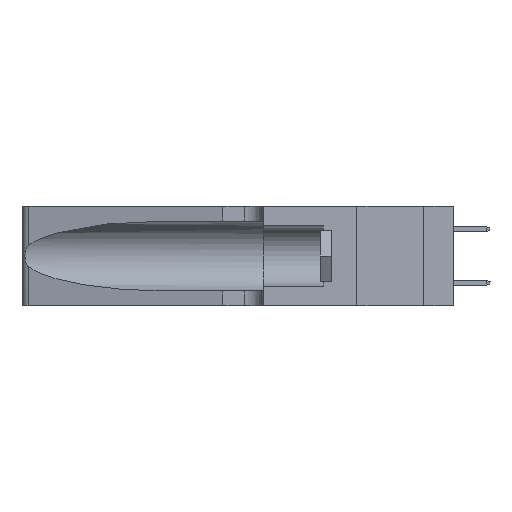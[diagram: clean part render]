
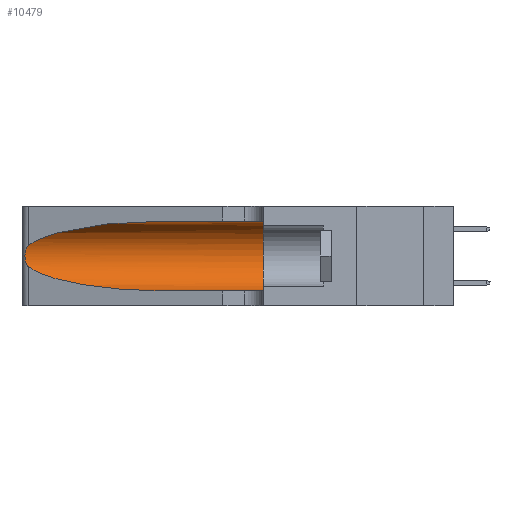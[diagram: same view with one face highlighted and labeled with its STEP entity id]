
A CAD part, left-side view. The second image highlights one B-rep face of the part: STEP entity #10479.
In plain terms, the highlighted cylindrical face has radius 3.308 mm (diameter 6.617 mm), a partial arc.
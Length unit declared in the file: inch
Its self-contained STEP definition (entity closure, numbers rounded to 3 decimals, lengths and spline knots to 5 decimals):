
#151 = CARTESIAN_POINT ( 'NONE',  ( 0.25789, 1.23486, 0.15765 ) ) ;
#358 = CYLINDRICAL_SURFACE ( 'NONE', #23111, 0.13025 ) ;
#1405 = CARTESIAN_POINT ( 'NONE',  ( 0.26018, 1.23835, 0.19895 ) ) ;
#1542 = CARTESIAN_POINT ( 'NONE',  ( 0.26017, 1.23833, 0.17102 ) ) ;
#2279 = CARTESIAN_POINT ( 'NONE',  ( 0.2373, 1.15595, 0.08982 ) ) ;
#2814 = DIRECTION ( 'NONE',  ( 0., -1., 0. ) ) ;
#2827 = CARTESIAN_POINT ( 'NONE',  ( 0.1305, 0.72297, 0.05475 ) ) ;
#3332 =( BOUNDED_CURVE ( )  B_SPLINE_CURVE ( 3, ( #8918, #2279, #21794, #2827 ),
 .UNSPECIFIED., .F., .T. ) 
 B_SPLINE_CURVE_WITH_KNOTS ( ( 4, 4 ),
 ( 3.44316, 4.71239 ),
 .UNSPECIFIED. ) 
 CURVE ( )  GEOMETRIC_REPRESENTATION_ITEM ( )  RATIONAL_B_SPLINE_CURVE ( ( 1., 0.87, 0.87, 1. ) ) 
 REPRESENTATION_ITEM ( '' )  );
#4428 = CARTESIAN_POINT ( 'NONE',  ( 0.25639, 1.23186, 0.15144 ) ) ;
#5728 = CARTESIAN_POINT ( 'NONE',  ( 0.1305, 0.72297, 0.31525 ) ) ;
#6187 =( BOUNDED_CURVE ( )  B_SPLINE_CURVE ( 3, ( #18186, #7313, #17913, #24366 ),
 .UNSPECIFIED., .F., .T. ) 
 B_SPLINE_CURVE_WITH_KNOTS ( ( 4, 4 ),
 ( 1.5708, 2.84003 ),
 .UNSPECIFIED. ) 
 CURVE ( )  GEOMETRIC_REPRESENTATION_ITEM ( )  RATIONAL_B_SPLINE_CURVE ( ( 1., 0.87, 0.87, 1. ) ) 
 REPRESENTATION_ITEM ( '' )  );
#6257 = CARTESIAN_POINT ( 'NONE',  ( 0.25555, 1.22994, 0.2215 ) ) ;
#6322 = B_SPLINE_CURVE_WITH_KNOTS ( 'NONE', 3,
 ( #25390, #6257, #20649, #23316, #20500, #1405, #9857, #18390, #1542, #25937, #151, #4428, #17109, #6814 ),
 .UNSPECIFIED., .F., .F.,
 ( 4, 2, 2, 2, 2, 2, 4 ),
 ( 0., 0.00027, 0.00053, 0.00107, 0.0016, 0.00187, 0.00214 ),
 .UNSPECIFIED. ) ;
#6324 = EDGE_CURVE ( 'NONE', #24706, #10597, #6322, .T. ) ;
#6612 = CARTESIAN_POINT ( 'NONE',  ( 0.1305, 1.61858, 0.185 ) ) ;
#6814 = CARTESIAN_POINT ( 'NONE',  ( 0.25487, 1.22718, 0.14631 ) ) ;
#7099 = EDGE_CURVE ( 'NONE', #10597, #18471, #3332, .T. ) ;
#7313 = CARTESIAN_POINT ( 'NONE',  ( 0.18966, 0.96281, 0.31525 ) ) ;
#7575 = CARTESIAN_POINT ( 'NONE',  ( 0.25487, 1.22718, 0.22369 ) ) ;
#8108 = VECTOR ( 'NONE', #2814, 39.37008 ) ;
#8449 = LINE ( 'NONE', #16953, #21588 ) ;
#8812 = DIRECTION ( 'NONE',  ( 0., 0., -1. ) ) ;
#8918 = CARTESIAN_POINT ( 'NONE',  ( 0.25487, 1.22718, 0.14631 ) ) ;
#9202 = CARTESIAN_POINT ( 'NONE',  ( 0.1305, 0.35, 0.31525 ) ) ;
#9857 = CARTESIAN_POINT ( 'NONE',  ( 0.26075, 1.23896, 0.19203 ) ) ;
#10479 = ADVANCED_FACE ( 'NONE', ( #19033 ), #358, .F. ) ;
#10597 = VERTEX_POINT ( 'NONE', #18006 ) ;
#10828 = EDGE_CURVE ( 'NONE', #14781, #13628, #20877, .T. ) ;
#11221 = CARTESIAN_POINT ( 'NONE',  ( 0.1305, 0.35, 0.185 ) ) ;
#12844 = CARTESIAN_POINT ( 'NONE',  ( 0.1305, 0.35, 0.05475 ) ) ;
#13628 = VERTEX_POINT ( 'NONE', #12844 ) ;
#14781 = VERTEX_POINT ( 'NONE', #9202 ) ;
#14929 = CARTESIAN_POINT ( 'NONE',  ( 0.1305, 0.72297, 0.05475 ) ) ;
#14930 = ORIENTED_EDGE ( 'NONE', *, *, #7099, .T. ) ;
#15316 = LINE ( 'NONE', #15461, #8108 ) ;
#15461 = CARTESIAN_POINT ( 'NONE',  ( 0.1305, 1.61858, 0.05475 ) ) ;
#16953 = CARTESIAN_POINT ( 'NONE',  ( 0.1305, 1.61858, 0.31525 ) ) ;
#17109 = CARTESIAN_POINT ( 'NONE',  ( 0.25555, 1.22993, 0.14849 ) ) ;
#17164 = ORIENTED_EDGE ( 'NONE', *, *, #6324, .T. ) ;
#17363 = DIRECTION ( 'NONE',  ( 0., 0., 1. ) ) ;
#17567 = EDGE_CURVE ( 'NONE', #18471, #13628, #15316, .T. ) ;
#17913 = CARTESIAN_POINT ( 'NONE',  ( 0.2373, 1.15595, 0.28018 ) ) ;
#18006 = CARTESIAN_POINT ( 'NONE',  ( 0.25487, 1.22718, 0.14631 ) ) ;
#18168 = AXIS2_PLACEMENT_3D ( 'NONE', #11221, #23702, #17363 ) ;
#18186 = CARTESIAN_POINT ( 'NONE',  ( 0.1305, 0.72297, 0.31525 ) ) ;
#18390 = CARTESIAN_POINT ( 'NONE',  ( 0.26075, 1.23896, 0.178 ) ) ;
#18471 = VERTEX_POINT ( 'NONE', #14929 ) ;
#18586 = ORIENTED_EDGE ( 'NONE', *, *, #27002, .F. ) ;
#19033 = FACE_OUTER_BOUND ( 'NONE', #24529, .T. ) ;
#20500 = CARTESIAN_POINT ( 'NONE',  ( 0.25854, 1.2359, 0.20912 ) ) ;
#20649 = CARTESIAN_POINT ( 'NONE',  ( 0.25639, 1.23184, 0.21858 ) ) ;
#20674 = ORIENTED_EDGE ( 'NONE', *, *, #10828, .F. ) ;
#20877 = CIRCLE ( 'NONE', #18168, 0.13025 ) ;
#21021 = VERTEX_POINT ( 'NONE', #5728 ) ;
#21588 = VECTOR ( 'NONE', #23714, 39.37008 ) ;
#21794 = CARTESIAN_POINT ( 'NONE',  ( 0.18966, 0.96281, 0.05475 ) ) ;
#21828 = ORIENTED_EDGE ( 'NONE', *, *, #17567, .T. ) ;
#23111 = AXIS2_PLACEMENT_3D ( 'NONE', #6612, #23653, #8812 ) ;
#23316 = CARTESIAN_POINT ( 'NONE',  ( 0.25787, 1.23484, 0.2124 ) ) ;
#23653 = DIRECTION ( 'NONE',  ( 0., -1., 0. ) ) ;
#23702 = DIRECTION ( 'NONE',  ( 0., 1., 0. ) ) ;
#23714 = DIRECTION ( 'NONE',  ( 0., -1., 0. ) ) ;
#24366 = CARTESIAN_POINT ( 'NONE',  ( 0.25487, 1.22718, 0.22369 ) ) ;
#24529 = EDGE_LOOP ( 'NONE', ( #24556, #17164, #14930, #21828, #20674, #18586 ) ) ;
#24556 = ORIENTED_EDGE ( 'NONE', *, *, #26660, .T. ) ;
#24706 = VERTEX_POINT ( 'NONE', #7575 ) ;
#25390 = CARTESIAN_POINT ( 'NONE',  ( 0.25487, 1.22718, 0.22369 ) ) ;
#25937 = CARTESIAN_POINT ( 'NONE',  ( 0.25856, 1.23593, 0.16098 ) ) ;
#26660 = EDGE_CURVE ( 'NONE', #21021, #24706, #6187, .T. ) ;
#27002 = EDGE_CURVE ( 'NONE', #21021, #14781, #8449, .T. ) ;
